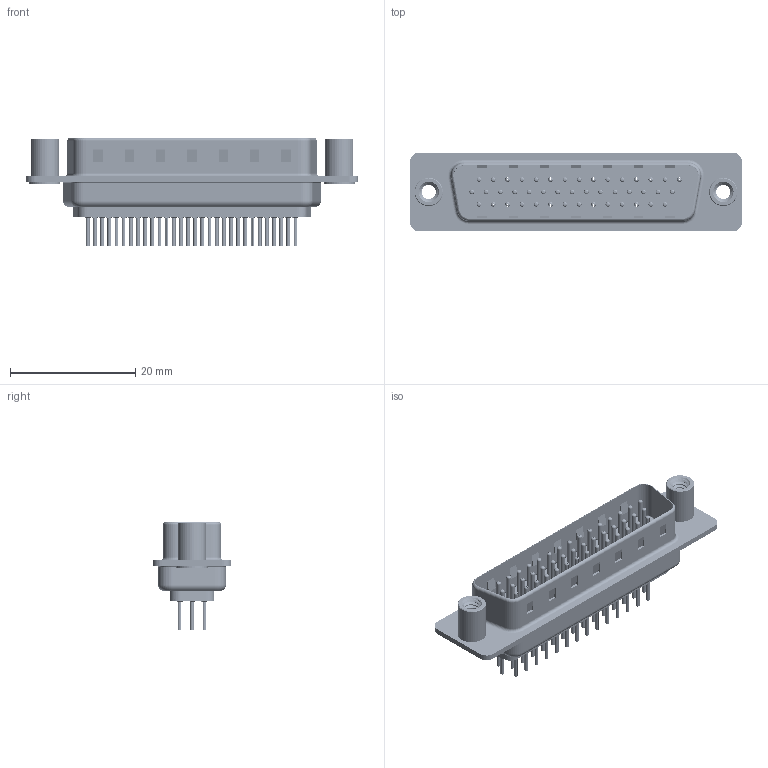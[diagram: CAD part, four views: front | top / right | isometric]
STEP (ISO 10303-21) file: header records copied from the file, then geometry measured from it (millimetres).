
FILE_DESCRIPTION (( 'STEP AP203' ), '1' );
FILE_NAME ('637-044-330-269.STEP', '2020-07-18T02:30:03', ( '' ), ( '' ), 'SwSTEP 2.0', 'SolidWorks 2020', '' );
FILE_SCHEMA (( 'CONFIG_CONTROL_DESIGN' ));
Length unit declared in the file: millimetre
Products named in the file (8): 637 Contact Row 3_30; 637 Shell Front_44 Contacts; 637 4-40 Threaded Standoff; 637 Contact Row 1_30; 637 Contact Row 2_30; 637-044-330-269; 637 Housing_44 Contacts; 637 Shell Rear_44 Contacts
Assembly tree (49 placements, depth 2):
  637-044-330-269
    637 Housing_44 Contacts
    637 Shell Front_44 Contacts
    637 Shell Rear_44 Contacts
    637 Contact Row 1_30  x15
    637 Contact Row 2_30  x15
    637 Contact Row 3_30  x14
    637 4-40 Threaded Standoff  x2
Bounding box: 53 x 12.6 x 17.25 mm (x, y, z)
Volume: 2732.6 mm3; surface area: 10232.5 mm2
Topology: 49 solids, 49 shells, 4810 faces, 12709 edges, 7834 vertices
Faces by surface type: cylinder 1793, torus 1326, plane 1229, cone 456, bspline 6
Entity records: 34117 total; most frequent: CARTESIAN_POINT 7649, DIRECTION 5527, ORIENTED_EDGE 4862, EDGE_CURVE 2431, AXIS2_PLACEMENT_3D 2232, VERTEX_POINT 1555, EDGE_LOOP 1216, CIRCLE 1195
